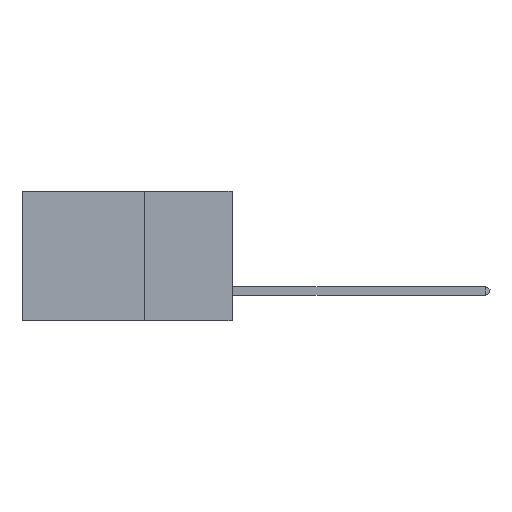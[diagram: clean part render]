
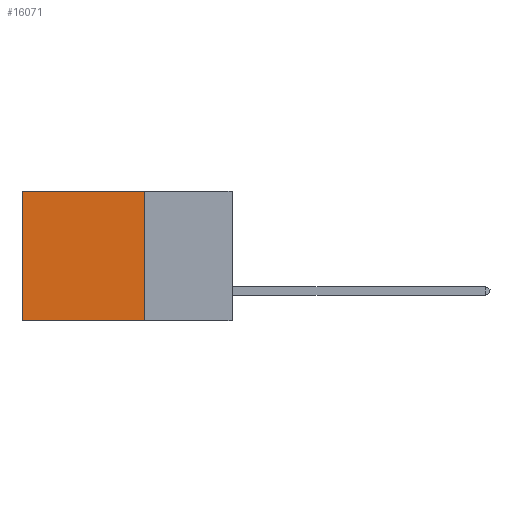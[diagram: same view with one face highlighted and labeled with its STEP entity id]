
A CAD part, left-side view. The second image highlights one B-rep face of the part: STEP entity #16071.
In plain terms, the highlighted planar face has unit normal (-1, 0, 0).
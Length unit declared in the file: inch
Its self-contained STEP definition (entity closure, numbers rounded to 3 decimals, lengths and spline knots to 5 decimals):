
#432 = ORIENTED_EDGE ( 'NONE', *, *, #6224, .T. ) ;
#1127 = EDGE_CURVE ( 'NONE', #15729, #6757, #3345, .T. ) ;
#2112 = DIRECTION ( 'NONE',  ( 0., 0., -1. ) ) ;
#3133 = DIRECTION ( 'NONE',  ( 0., 1., 0. ) ) ;
#3345 = LINE ( 'NONE', #9576, #9189 ) ;
#5537 = DIRECTION ( 'NONE',  ( 1., 0., 0. ) ) ;
#5587 = EDGE_LOOP ( 'NONE', ( #432, #15085, #7761, #8332 ) ) ;
#6224 = EDGE_CURVE ( 'NONE', #10643, #12130, #10986, .T. ) ;
#6319 = CARTESIAN_POINT ( 'NONE',  ( 0.2875, 0.25, 0. ) ) ;
#6430 = EDGE_CURVE ( 'NONE', #6757, #12130, #15323, .T. ) ;
#6701 = CARTESIAN_POINT ( 'NONE',  ( 0.2875, 0.25, -0.37 ) ) ;
#6757 = VERTEX_POINT ( 'NONE', #14495 ) ;
#7458 = VECTOR ( 'NONE', #10825, 39.37008 ) ;
#7500 = CARTESIAN_POINT ( 'NONE',  ( 0.2875, 0.25, 0. ) ) ;
#7761 = ORIENTED_EDGE ( 'NONE', *, *, #1127, .F. ) ;
#8332 = ORIENTED_EDGE ( 'NONE', *, *, #13291, .T. ) ;
#9189 = VECTOR ( 'NONE', #2112, 39.37008 ) ;
#9576 = CARTESIAN_POINT ( 'NONE',  ( 0.2875, 0.25, 0. ) ) ;
#10643 = VERTEX_POINT ( 'NONE', #13908 ) ;
#10735 = DIRECTION ( 'NONE',  ( 0., 0., -1. ) ) ;
#10825 = DIRECTION ( 'NONE',  ( 0., 0., -1. ) ) ;
#10986 = LINE ( 'NONE', #15783, #7458 ) ;
#11028 = FACE_OUTER_BOUND ( 'NONE', #5587, .T. ) ;
#11750 = VECTOR ( 'NONE', #12410, 39.37008 ) ;
#11797 = CARTESIAN_POINT ( 'NONE',  ( 0.2875, 0.25, 0. ) ) ;
#11989 = VECTOR ( 'NONE', #3133, 39.37008 ) ;
#12130 = VERTEX_POINT ( 'NONE', #14728 ) ;
#12410 = DIRECTION ( 'NONE',  ( 0., 1., 0. ) ) ;
#12560 = LINE ( 'NONE', #7500, #11750 ) ;
#13291 = EDGE_CURVE ( 'NONE', #15729, #10643, #12560, .T. ) ;
#13433 = AXIS2_PLACEMENT_3D ( 'NONE', #11797, #5537, #10735 ) ;
#13908 = CARTESIAN_POINT ( 'NONE',  ( 0.2875, 0.6, 0. ) ) ;
#14495 = CARTESIAN_POINT ( 'NONE',  ( 0.2875, 0.25, -0.37 ) ) ;
#14521 = PLANE ( 'NONE',  #13433 ) ;
#14728 = CARTESIAN_POINT ( 'NONE',  ( 0.2875, 0.6, -0.37 ) ) ;
#15085 = ORIENTED_EDGE ( 'NONE', *, *, #6430, .F. ) ;
#15323 = LINE ( 'NONE', #6701, #11989 ) ;
#15729 = VERTEX_POINT ( 'NONE', #6319 ) ;
#15783 = CARTESIAN_POINT ( 'NONE',  ( 0.2875, 0.6, 0. ) ) ;
#16071 = ADVANCED_FACE ( 'NONE', ( #11028 ), #14521, .F. ) ;
